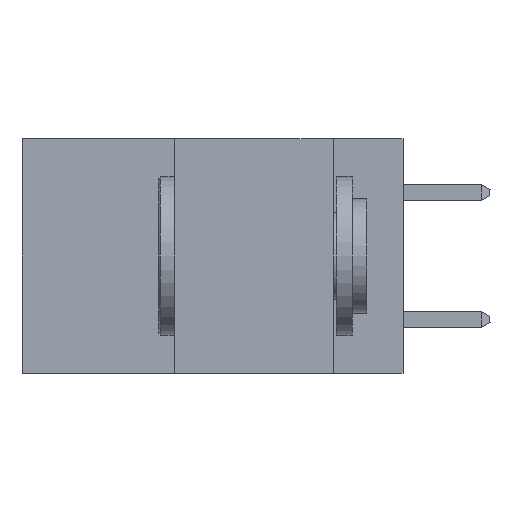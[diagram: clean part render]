
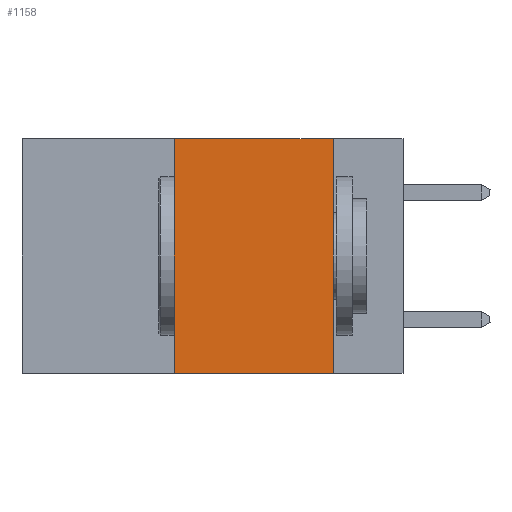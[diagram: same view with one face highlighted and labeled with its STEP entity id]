
A CAD part, left-side view. The second image highlights one B-rep face of the part: STEP entity #1158.
In plain terms, the highlighted planar face has unit normal (-1, 0, 0).
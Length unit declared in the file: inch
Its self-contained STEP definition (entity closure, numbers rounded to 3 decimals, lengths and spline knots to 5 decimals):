
#81 = CARTESIAN_POINT ( 'NONE',  ( 0., 0.6, 0. ) ) ;
#258 = VECTOR ( 'NONE', #8594, 39.37008 ) ;
#1103 = ORIENTED_EDGE ( 'NONE', *, *, #17400, .F. ) ;
#1158 = ADVANCED_FACE ( 'NONE', ( #5766 ), #7023, .F. ) ;
#1179 = VERTEX_POINT ( 'NONE', #2635 ) ;
#1207 = DIRECTION ( 'NONE',  ( 0., 0., -1. ) ) ;
#1804 = ORIENTED_EDGE ( 'NONE', *, *, #7736, .F. ) ;
#2190 = AXIS2_PLACEMENT_3D ( 'NONE', #14299, #17197, #1207 ) ;
#2635 = CARTESIAN_POINT ( 'NONE',  ( 0., 0.11, 0. ) ) ;
#2902 = VECTOR ( 'NONE', #13774, 39.37008 ) ;
#2936 = EDGE_CURVE ( 'NONE', #8078, #13057, #8817, .T. ) ;
#4694 = VECTOR ( 'NONE', #7816, 39.37008 ) ;
#5460 = CARTESIAN_POINT ( 'NONE',  ( 0., 0.36, -0.37 ) ) ;
#5766 = FACE_OUTER_BOUND ( 'NONE', #14320, .T. ) ;
#6126 = CARTESIAN_POINT ( 'NONE',  ( 0., 0.36, 0. ) ) ;
#6194 = EDGE_CURVE ( 'NONE', #18054, #1179, #18222, .T. ) ;
#7023 = PLANE ( 'NONE',  #2190 ) ;
#7736 = EDGE_CURVE ( 'NONE', #1179, #13057, #10657, .T. ) ;
#7816 = DIRECTION ( 'NONE',  ( 0., -1., 0. ) ) ;
#8078 = VERTEX_POINT ( 'NONE', #5460 ) ;
#8102 = LINE ( 'NONE', #13425, #18778 ) ;
#8594 = DIRECTION ( 'NONE',  ( 0., -1., 0. ) ) ;
#8817 = LINE ( 'NONE', #10748, #4694 ) ;
#9569 = ORIENTED_EDGE ( 'NONE', *, *, #2936, .T. ) ;
#10657 = LINE ( 'NONE', #10829, #2902 ) ;
#10748 = CARTESIAN_POINT ( 'NONE',  ( 0., 0.6, -0.37 ) ) ;
#10829 = CARTESIAN_POINT ( 'NONE',  ( 0., 0.11, 0. ) ) ;
#13057 = VERTEX_POINT ( 'NONE', #18046 ) ;
#13425 = CARTESIAN_POINT ( 'NONE',  ( 0., 0.36, 0. ) ) ;
#13774 = DIRECTION ( 'NONE',  ( 0., 0., -1. ) ) ;
#14299 = CARTESIAN_POINT ( 'NONE',  ( 0., 0.6, 0. ) ) ;
#14320 = EDGE_LOOP ( 'NONE', ( #1804, #15435, #1103, #9569 ) ) ;
#14950 = DIRECTION ( 'NONE',  ( 0., 0., 1. ) ) ;
#15435 = ORIENTED_EDGE ( 'NONE', *, *, #6194, .F. ) ;
#17197 = DIRECTION ( 'NONE',  ( 1., 0., 0. ) ) ;
#17400 = EDGE_CURVE ( 'NONE', #8078, #18054, #8102, .T. ) ;
#18046 = CARTESIAN_POINT ( 'NONE',  ( 0., 0.11, -0.37 ) ) ;
#18054 = VERTEX_POINT ( 'NONE', #6126 ) ;
#18222 = LINE ( 'NONE', #81, #258 ) ;
#18778 = VECTOR ( 'NONE', #14950, 39.37008 ) ;
